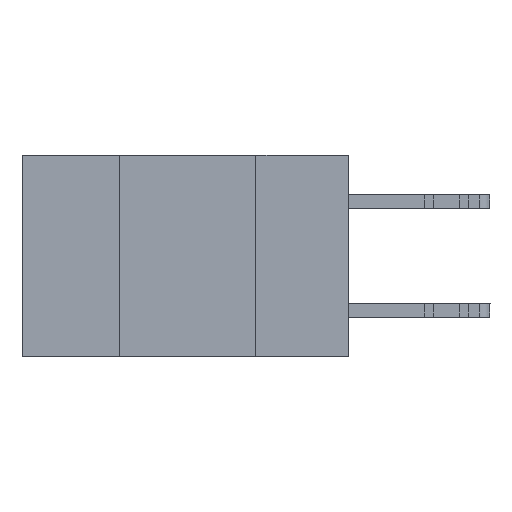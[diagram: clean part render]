
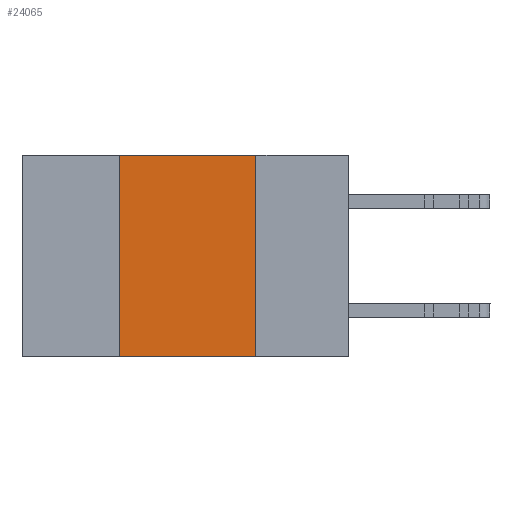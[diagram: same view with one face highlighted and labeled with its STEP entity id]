
A CAD part, left-side view. The second image highlights one B-rep face of the part: STEP entity #24065.
In plain terms, the highlighted planar face has unit normal (-1, 0, 0).
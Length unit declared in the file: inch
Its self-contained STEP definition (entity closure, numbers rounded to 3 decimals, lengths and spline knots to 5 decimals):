
#1220 = VECTOR ( 'NONE', #13467, 39.37008 ) ;
#1569 = PLANE ( 'NONE',  #23823 ) ;
#2055 = EDGE_CURVE ( 'NONE', #20797, #5129, #10638, .T. ) ;
#2960 = VERTEX_POINT ( 'NONE', #24655 ) ;
#3357 = CARTESIAN_POINT ( 'NONE',  ( 0., 0.6, -0.37 ) ) ;
#4001 = ORIENTED_EDGE ( 'NONE', *, *, #11139, .T. ) ;
#5129 = VERTEX_POINT ( 'NONE', #21451 ) ;
#6505 = VECTOR ( 'NONE', #21185, 39.37008 ) ;
#7615 = CARTESIAN_POINT ( 'NONE',  ( 0., 0.17, 0. ) ) ;
#8925 = EDGE_LOOP ( 'NONE', ( #12333, #19301, #12686, #4001 ) ) ;
#9055 = CARTESIAN_POINT ( 'NONE',  ( 0., 0.6, 0. ) ) ;
#10638 = LINE ( 'NONE', #23735, #1220 ) ;
#11139 = EDGE_CURVE ( 'NONE', #20797, #2960, #20761, .T. ) ;
#11345 = DIRECTION ( 'NONE',  ( 1., 0., 0. ) ) ;
#11823 = EDGE_CURVE ( 'NONE', #17993, #2960, #14850, .T. ) ;
#12033 = LINE ( 'NONE', #23698, #6505 ) ;
#12333 = ORIENTED_EDGE ( 'NONE', *, *, #11823, .F. ) ;
#12686 = ORIENTED_EDGE ( 'NONE', *, *, #2055, .F. ) ;
#12854 = VECTOR ( 'NONE', #18262, 39.37008 ) ;
#13467 = DIRECTION ( 'NONE',  ( 0., 0., 1. ) ) ;
#13836 = CARTESIAN_POINT ( 'NONE',  ( 0., 0.17, 0. ) ) ;
#13851 = CARTESIAN_POINT ( 'NONE',  ( 0., 0.42, -0.37 ) ) ;
#14850 = LINE ( 'NONE', #13836, #24270 ) ;
#16625 = DIRECTION ( 'NONE',  ( 0., 0., -1. ) ) ;
#17993 = VERTEX_POINT ( 'NONE', #7615 ) ;
#18262 = DIRECTION ( 'NONE',  ( 0., -1., 0. ) ) ;
#19206 = DIRECTION ( 'NONE',  ( 0., 0., -1. ) ) ;
#19301 = ORIENTED_EDGE ( 'NONE', *, *, #20448, .F. ) ;
#20448 = EDGE_CURVE ( 'NONE', #5129, #17993, #12033, .T. ) ;
#20761 = LINE ( 'NONE', #3357, #12854 ) ;
#20797 = VERTEX_POINT ( 'NONE', #13851 ) ;
#21185 = DIRECTION ( 'NONE',  ( 0., -1., 0. ) ) ;
#21451 = CARTESIAN_POINT ( 'NONE',  ( 0., 0.42, 0. ) ) ;
#23698 = CARTESIAN_POINT ( 'NONE',  ( 0., 0.6, 0. ) ) ;
#23735 = CARTESIAN_POINT ( 'NONE',  ( 0., 0.42, 0. ) ) ;
#23823 = AXIS2_PLACEMENT_3D ( 'NONE', #9055, #11345, #19206 ) ;
#24065 = ADVANCED_FACE ( 'NONE', ( #27403 ), #1569, .F. ) ;
#24270 = VECTOR ( 'NONE', #16625, 39.37008 ) ;
#24655 = CARTESIAN_POINT ( 'NONE',  ( 0., 0.17, -0.37 ) ) ;
#27403 = FACE_OUTER_BOUND ( 'NONE', #8925, .T. ) ;
